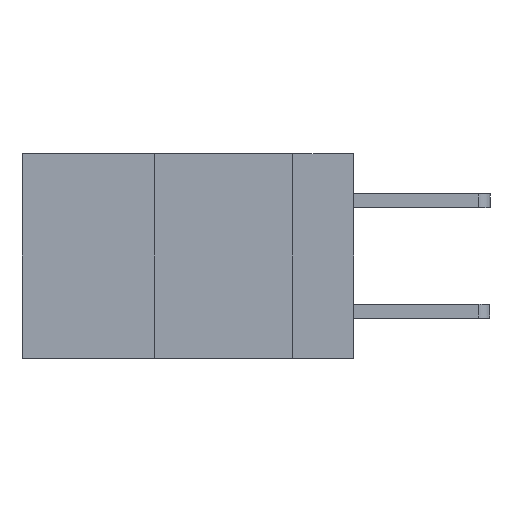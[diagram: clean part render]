
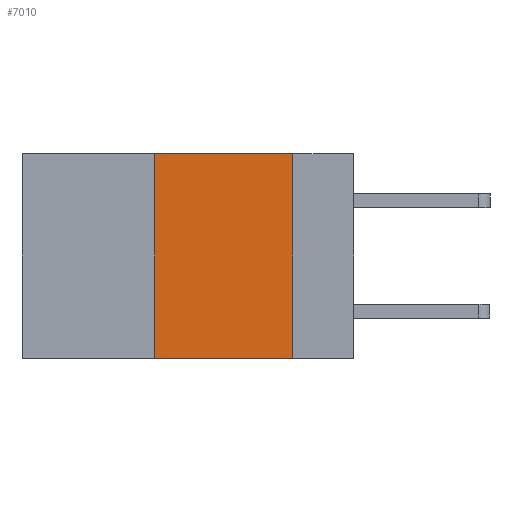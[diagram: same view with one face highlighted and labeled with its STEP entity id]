
A CAD part, left-side view. The second image highlights one B-rep face of the part: STEP entity #7010.
In plain terms, the highlighted planar face has unit normal (-1, 0, 0).
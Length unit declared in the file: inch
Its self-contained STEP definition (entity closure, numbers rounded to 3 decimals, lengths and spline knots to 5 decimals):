
#11 = CARTESIAN_POINT ( 'NONE',  ( 0., 0.36, 0. ) ) ;
#63 = EDGE_CURVE ( 'NONE', #5407, #2711, #3647, .T. ) ;
#93 = VERTEX_POINT ( 'NONE', #3267 ) ;
#385 = CARTESIAN_POINT ( 'NONE',  ( 0., 0.36, 0. ) ) ;
#996 = DIRECTION ( 'NONE',  ( 0., -1., 0. ) ) ;
#1596 = DIRECTION ( 'NONE',  ( 0., -1., 0. ) ) ;
#1660 = LINE ( 'NONE', #5062, #5096 ) ;
#1932 = CARTESIAN_POINT ( 'NONE',  ( 0., 0.6, -0.37 ) ) ;
#2270 = VECTOR ( 'NONE', #10417, 39.37008 ) ;
#2711 = VERTEX_POINT ( 'NONE', #11 ) ;
#3267 = CARTESIAN_POINT ( 'NONE',  ( 0., 0.11, -0.37 ) ) ;
#3647 = LINE ( 'NONE', #385, #2270 ) ;
#4563 = ORIENTED_EDGE ( 'NONE', *, *, #7144, .T. ) ;
#4835 = PLANE ( 'NONE',  #4881 ) ;
#4881 = AXIS2_PLACEMENT_3D ( 'NONE', #9128, #9059, #8292 ) ;
#5062 = CARTESIAN_POINT ( 'NONE',  ( 0., 0.6, 0. ) ) ;
#5096 = VECTOR ( 'NONE', #1596, 39.37008 ) ;
#5338 = CARTESIAN_POINT ( 'NONE',  ( 0., 0.36, -0.37 ) ) ;
#5407 = VERTEX_POINT ( 'NONE', #5338 ) ;
#5449 = DIRECTION ( 'NONE',  ( 0., 0., -1. ) ) ;
#5670 = FACE_OUTER_BOUND ( 'NONE', #9934, .T. ) ;
#5972 = ORIENTED_EDGE ( 'NONE', *, *, #8114, .F. ) ;
#6020 = ORIENTED_EDGE ( 'NONE', *, *, #6957, .F. ) ;
#6485 = CARTESIAN_POINT ( 'NONE',  ( 0., 0.11, 0. ) ) ;
#6957 = EDGE_CURVE ( 'NONE', #7706, #93, #10575, .T. ) ;
#7010 = ADVANCED_FACE ( 'NONE', ( #5670 ), #4835, .F. ) ;
#7144 = EDGE_CURVE ( 'NONE', #5407, #93, #7965, .T. ) ;
#7706 = VERTEX_POINT ( 'NONE', #6485 ) ;
#7898 = VECTOR ( 'NONE', #5449, 39.37008 ) ;
#7965 = LINE ( 'NONE', #1932, #10593 ) ;
#8114 = EDGE_CURVE ( 'NONE', #2711, #7706, #1660, .T. ) ;
#8292 = DIRECTION ( 'NONE',  ( 0., 0., -1. ) ) ;
#8467 = ORIENTED_EDGE ( 'NONE', *, *, #63, .F. ) ;
#9059 = DIRECTION ( 'NONE',  ( 1., 0., 0. ) ) ;
#9128 = CARTESIAN_POINT ( 'NONE',  ( 0., 0.6, 0. ) ) ;
#9934 = EDGE_LOOP ( 'NONE', ( #6020, #5972, #8467, #4563 ) ) ;
#10417 = DIRECTION ( 'NONE',  ( 0., 0., 1. ) ) ;
#10474 = CARTESIAN_POINT ( 'NONE',  ( 0., 0.11, 0. ) ) ;
#10575 = LINE ( 'NONE', #10474, #7898 ) ;
#10593 = VECTOR ( 'NONE', #996, 39.37008 ) ;
